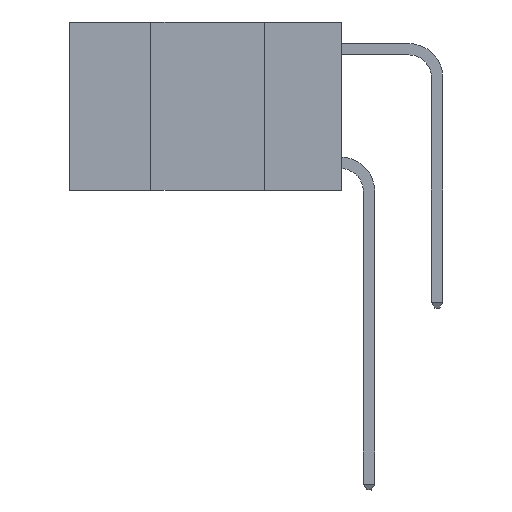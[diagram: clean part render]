
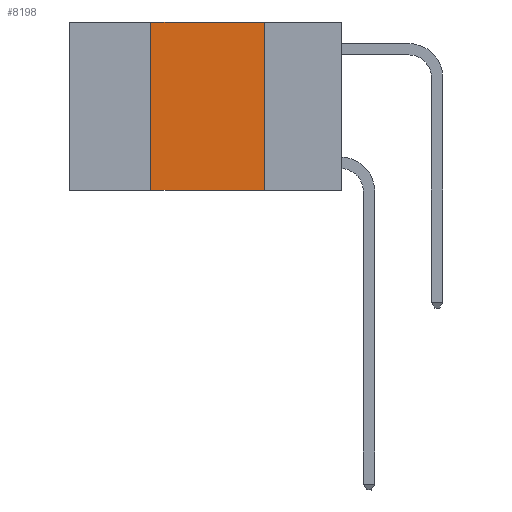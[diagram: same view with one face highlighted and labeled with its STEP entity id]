
A CAD part, left-side view. The second image highlights one B-rep face of the part: STEP entity #8198.
In plain terms, the highlighted planar face has unit normal (-1, 0, 0).
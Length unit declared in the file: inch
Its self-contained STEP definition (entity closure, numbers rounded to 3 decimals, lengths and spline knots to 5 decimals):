
#88 = PLANE ( 'NONE',  #9759 ) ;
#171 = ORIENTED_EDGE ( 'NONE', *, *, #4434, .F. ) ;
#177 = ORIENTED_EDGE ( 'NONE', *, *, #9501, .F. ) ;
#272 = EDGE_LOOP ( 'NONE', ( #171, #177, #4839, #9396 ) ) ;
#829 = LINE ( 'NONE', #9143, #8605 ) ;
#854 = CARTESIAN_POINT ( 'NONE',  ( 0., 0.42, 0. ) ) ;
#2227 = VERTEX_POINT ( 'NONE', #4474 ) ;
#2259 = EDGE_CURVE ( 'NONE', #10130, #5726, #4022, .T. ) ;
#2434 = DIRECTION ( 'NONE',  ( 0., 0., 1. ) ) ;
#4022 = LINE ( 'NONE', #854, #9302 ) ;
#4072 = VECTOR ( 'NONE', #8629, 39.37008 ) ;
#4162 = DIRECTION ( 'NONE',  ( 0., 0., -1. ) ) ;
#4365 = VECTOR ( 'NONE', #6565, 39.37008 ) ;
#4434 = EDGE_CURVE ( 'NONE', #8385, #2227, #8367, .T. ) ;
#4474 = CARTESIAN_POINT ( 'NONE',  ( 0., 0.17, -0.37 ) ) ;
#4839 = ORIENTED_EDGE ( 'NONE', *, *, #2259, .F. ) ;
#4905 = CARTESIAN_POINT ( 'NONE',  ( 0., 0.17, 0. ) ) ;
#5055 = DIRECTION ( 'NONE',  ( 0., -1., 0. ) ) ;
#5067 = FACE_OUTER_BOUND ( 'NONE', #272, .T. ) ;
#5726 = VERTEX_POINT ( 'NONE', #7956 ) ;
#6565 = DIRECTION ( 'NONE',  ( 0., 0., -1. ) ) ;
#7366 = DIRECTION ( 'NONE',  ( 1., 0., 0. ) ) ;
#7956 = CARTESIAN_POINT ( 'NONE',  ( 0., 0.42, 0. ) ) ;
#8133 = CARTESIAN_POINT ( 'NONE',  ( 0., 0.17, 0. ) ) ;
#8198 = ADVANCED_FACE ( 'NONE', ( #5067 ), #88, .F. ) ;
#8367 = LINE ( 'NONE', #8133, #4365 ) ;
#8385 = VERTEX_POINT ( 'NONE', #4905 ) ;
#8432 = EDGE_CURVE ( 'NONE', #10130, #2227, #10143, .T. ) ;
#8605 = VECTOR ( 'NONE', #5055, 39.37008 ) ;
#8629 = DIRECTION ( 'NONE',  ( 0., -1., 0. ) ) ;
#8698 = CARTESIAN_POINT ( 'NONE',  ( 0., 0.6, -0.37 ) ) ;
#8987 = CARTESIAN_POINT ( 'NONE',  ( 0., 0.42, -0.37 ) ) ;
#9143 = CARTESIAN_POINT ( 'NONE',  ( 0., 0.6, 0. ) ) ;
#9302 = VECTOR ( 'NONE', #2434, 39.37008 ) ;
#9396 = ORIENTED_EDGE ( 'NONE', *, *, #8432, .T. ) ;
#9501 = EDGE_CURVE ( 'NONE', #5726, #8385, #829, .T. ) ;
#9759 = AXIS2_PLACEMENT_3D ( 'NONE', #10676, #7366, #4162 ) ;
#10130 = VERTEX_POINT ( 'NONE', #8987 ) ;
#10143 = LINE ( 'NONE', #8698, #4072 ) ;
#10676 = CARTESIAN_POINT ( 'NONE',  ( 0., 0.6, 0. ) ) ;
